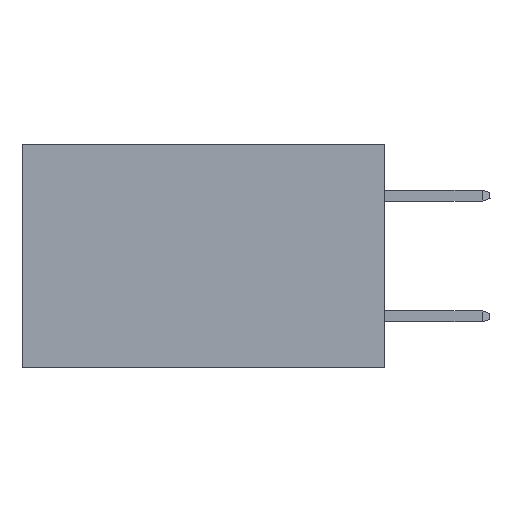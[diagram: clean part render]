
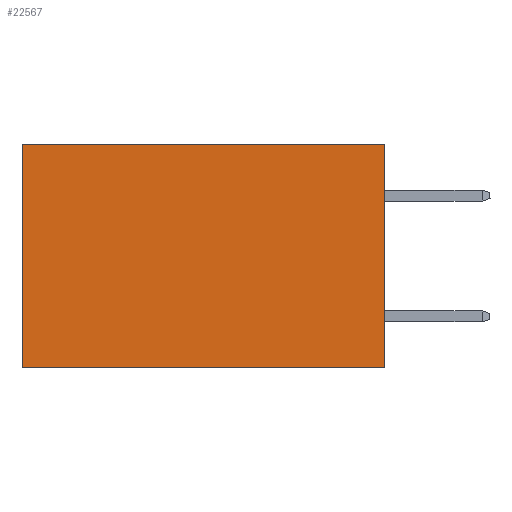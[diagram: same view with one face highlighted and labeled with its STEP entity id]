
A CAD part, left-side view. The second image highlights one B-rep face of the part: STEP entity #22567.
In plain terms, the highlighted planar face has unit normal (-1, 0, 0).
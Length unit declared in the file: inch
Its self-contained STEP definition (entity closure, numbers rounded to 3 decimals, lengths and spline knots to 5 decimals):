
#168 = ORIENTED_EDGE ( 'NONE', *, *, #24107, .F. ) ;
#1053 = VERTEX_POINT ( 'NONE', #2769 ) ;
#1591 = CARTESIAN_POINT ( 'NONE',  ( 0.298, 0.6, 0. ) ) ;
#1832 = DIRECTION ( 'NONE',  ( 1., 0., 0. ) ) ;
#2326 = EDGE_CURVE ( 'NONE', #25047, #1053, #18962, .T. ) ;
#2769 = CARTESIAN_POINT ( 'NONE',  ( 0.298, 0.6, 0. ) ) ;
#2773 = FACE_OUTER_BOUND ( 'NONE', #16730, .T. ) ;
#3654 = DIRECTION ( 'NONE',  ( 0., 0., -1. ) ) ;
#5001 = ORIENTED_EDGE ( 'NONE', *, *, #2326, .T. ) ;
#5511 = CARTESIAN_POINT ( 'NONE',  ( 0.298, 0.6, -0.37 ) ) ;
#6655 = CARTESIAN_POINT ( 'NONE',  ( 0.298, 0., 0. ) ) ;
#7093 = DIRECTION ( 'NONE',  ( 0., 1., 0. ) ) ;
#7467 = VERTEX_POINT ( 'NONE', #5511 ) ;
#7898 = VECTOR ( 'NONE', #9789, 39.37008 ) ;
#8652 = AXIS2_PLACEMENT_3D ( 'NONE', #13915, #1832, #15956 ) ;
#8661 = DIRECTION ( 'NONE',  ( 0., 0., -1. ) ) ;
#8892 = VECTOR ( 'NONE', #7093, 39.37008 ) ;
#8904 = EDGE_CURVE ( 'NONE', #22559, #7467, #19251, .T. ) ;
#9789 = DIRECTION ( 'NONE',  ( 0., 1., 0. ) ) ;
#9857 = PLANE ( 'NONE',  #8652 ) ;
#10969 = EDGE_CURVE ( 'NONE', #1053, #7467, #23472, .T. ) ;
#11815 = ORIENTED_EDGE ( 'NONE', *, *, #8904, .F. ) ;
#13915 = CARTESIAN_POINT ( 'NONE',  ( 0.298, 0., 0. ) ) ;
#14351 = CARTESIAN_POINT ( 'NONE',  ( 0.298, 0., 0. ) ) ;
#15956 = DIRECTION ( 'NONE',  ( 0., 0., -1. ) ) ;
#16277 = LINE ( 'NONE', #6655, #16909 ) ;
#16730 = EDGE_LOOP ( 'NONE', ( #24273, #11815, #168, #5001 ) ) ;
#16909 = VECTOR ( 'NONE', #8661, 39.37008 ) ;
#18406 = CARTESIAN_POINT ( 'NONE',  ( 0.298, 0., 0. ) ) ;
#18962 = LINE ( 'NONE', #14351, #8892 ) ;
#19251 = LINE ( 'NONE', #19836, #7898 ) ;
#19836 = CARTESIAN_POINT ( 'NONE',  ( 0.298, 0., -0.37 ) ) ;
#19899 = CARTESIAN_POINT ( 'NONE',  ( 0.298, 0., -0.37 ) ) ;
#22559 = VERTEX_POINT ( 'NONE', #19899 ) ;
#22567 = ADVANCED_FACE ( 'NONE', ( #2773 ), #9857, .F. ) ;
#22879 = VECTOR ( 'NONE', #3654, 39.37008 ) ;
#23472 = LINE ( 'NONE', #1591, #22879 ) ;
#24107 = EDGE_CURVE ( 'NONE', #25047, #22559, #16277, .T. ) ;
#24273 = ORIENTED_EDGE ( 'NONE', *, *, #10969, .T. ) ;
#25047 = VERTEX_POINT ( 'NONE', #18406 ) ;
